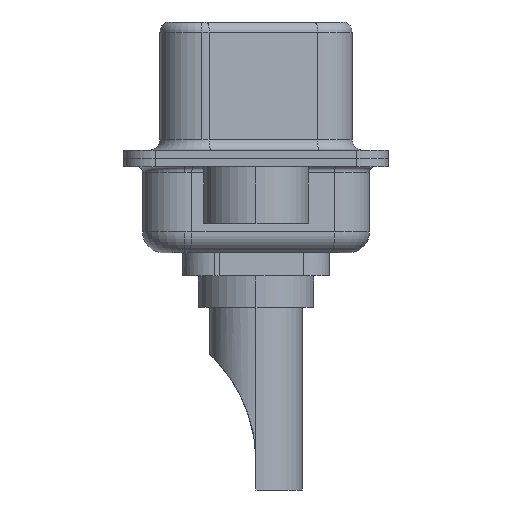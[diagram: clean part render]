
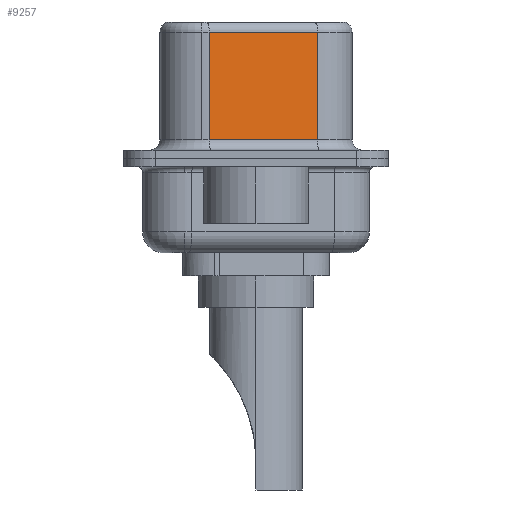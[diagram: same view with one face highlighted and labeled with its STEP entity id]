
A CAD part, left-side view. The second image highlights one B-rep face of the part: STEP entity #9257.
In plain terms, the highlighted planar face has unit normal (-0.985, -0.174, 0).
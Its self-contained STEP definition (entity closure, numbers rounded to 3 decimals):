
#277 = CARTESIAN_POINT ( 'NONE',  ( 4.585, -2.927, 6.02 ) ) ;
#332 = EDGE_CURVE ( 'NONE', #1287, #7783, #7735, .T. ) ;
#676 = VERTEX_POINT ( 'NONE', #18218 ) ;
#1287 = VERTEX_POINT ( 'NONE', #16404 ) ;
#1683 = ORIENTED_EDGE ( 'NONE', *, *, #332, .T. ) ;
#1970 = DIRECTION ( 'NONE',  ( 0., 0., -1. ) ) ;
#2087 = DIRECTION ( 'NONE',  ( 0., 0., -1. ) ) ;
#2290 = LINE ( 'NONE', #11760, #10654 ) ;
#3674 = VECTOR ( 'NONE', #12449, 1000. ) ;
#5030 = VERTEX_POINT ( 'NONE', #5274 ) ;
#5274 = CARTESIAN_POINT ( 'NONE',  ( 4.585, -2.927, 0.9 ) ) ;
#5435 = ORIENTED_EDGE ( 'NONE', *, *, #19335, .F. ) ;
#5822 = CARTESIAN_POINT ( 'NONE',  ( 3.675, 2.233, 0.9 ) ) ;
#7399 = PLANE ( 'NONE',  #11292 ) ;
#7420 = VECTOR ( 'NONE', #1970, 1000. ) ;
#7735 = LINE ( 'NONE', #9889, #19675 ) ;
#7783 = VERTEX_POINT ( 'NONE', #5822 ) ;
#9257 = ADVANCED_FACE ( 'NONE', ( #9724 ), #7399, .F. ) ;
#9572 = CARTESIAN_POINT ( 'NONE',  ( 4.585, -2.927, 6.52 ) ) ;
#9724 = FACE_OUTER_BOUND ( 'NONE', #14566, .T. ) ;
#9742 = ORIENTED_EDGE ( 'NONE', *, *, #10088, .T. ) ;
#9889 = CARTESIAN_POINT ( 'NONE',  ( 3.675, 2.233, 6.52 ) ) ;
#10088 = EDGE_CURVE ( 'NONE', #7783, #5030, #2290, .T. ) ;
#10107 = DIRECTION ( 'NONE',  ( 0.174, -0.985, 0. ) ) ;
#10558 = CARTESIAN_POINT ( 'NONE',  ( 4.585, -2.927, 6.52 ) ) ;
#10654 = VECTOR ( 'NONE', #10107, 1000. ) ;
#11292 = AXIS2_PLACEMENT_3D ( 'NONE', #10558, #18384, #12029 ) ;
#11760 = CARTESIAN_POINT ( 'NONE',  ( 4.585, -2.927, 0.9 ) ) ;
#12029 = DIRECTION ( 'NONE',  ( -0.174, 0.985, 0. ) ) ;
#12424 = EDGE_CURVE ( 'NONE', #676, #1287, #14220, .T. ) ;
#12449 = DIRECTION ( 'NONE',  ( -0.174, 0.985, 0. ) ) ;
#13475 = ORIENTED_EDGE ( 'NONE', *, *, #12424, .T. ) ;
#14220 = LINE ( 'NONE', #277, #3674 ) ;
#14566 = EDGE_LOOP ( 'NONE', ( #5435, #13475, #1683, #9742 ) ) ;
#16404 = CARTESIAN_POINT ( 'NONE',  ( 3.675, 2.233, 6.02 ) ) ;
#16538 = LINE ( 'NONE', #9572, #7420 ) ;
#18218 = CARTESIAN_POINT ( 'NONE',  ( 4.585, -2.927, 6.02 ) ) ;
#18384 = DIRECTION ( 'NONE',  ( 0.985, 0.174, 0. ) ) ;
#19335 = EDGE_CURVE ( 'NONE', #676, #5030, #16538, .T. ) ;
#19675 = VECTOR ( 'NONE', #2087, 1000. ) ;
